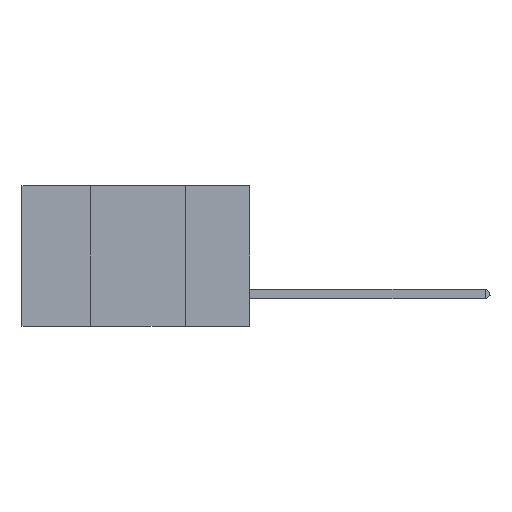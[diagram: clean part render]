
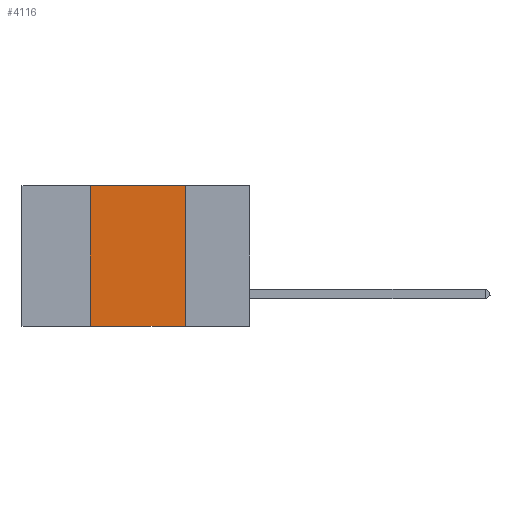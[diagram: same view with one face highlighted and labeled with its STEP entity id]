
A CAD part, left-side view. The second image highlights one B-rep face of the part: STEP entity #4116.
In plain terms, the highlighted planar face has unit normal (-1, 0, 0).
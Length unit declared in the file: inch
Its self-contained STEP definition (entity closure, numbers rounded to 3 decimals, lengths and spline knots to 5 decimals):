
#450 = EDGE_CURVE ( 'NONE', #1545, #4251, #6222, .T. ) ;
#472 = CARTESIAN_POINT ( 'NONE',  ( 0., 0.6, 0. ) ) ;
#520 = VECTOR ( 'NONE', #3350, 39.37008 ) ;
#592 = ORIENTED_EDGE ( 'NONE', *, *, #7883, .F. ) ;
#725 = VERTEX_POINT ( 'NONE', #2009 ) ;
#1063 = DIRECTION ( 'NONE',  ( 0., -1., 0. ) ) ;
#1291 = EDGE_LOOP ( 'NONE', ( #2982, #592, #4807, #7257 ) ) ;
#1545 = VERTEX_POINT ( 'NONE', #9071 ) ;
#2009 = CARTESIAN_POINT ( 'NONE',  ( 0., 0.17, -0.37 ) ) ;
#2027 = EDGE_CURVE ( 'NONE', #1545, #725, #5372, .T. ) ;
#2056 = AXIS2_PLACEMENT_3D ( 'NONE', #472, #8594, #6289 ) ;
#2134 = CARTESIAN_POINT ( 'NONE',  ( 0., 0.42, 0. ) ) ;
#2360 = EDGE_CURVE ( 'NONE', #4286, #725, #6974, .T. ) ;
#2982 = ORIENTED_EDGE ( 'NONE', *, *, #2360, .F. ) ;
#3350 = DIRECTION ( 'NONE',  ( 0., -1., 0. ) ) ;
#4076 = CARTESIAN_POINT ( 'NONE',  ( 0., 0.6, -0.37 ) ) ;
#4116 = ADVANCED_FACE ( 'NONE', ( #7621 ), #5554, .F. ) ;
#4251 = VERTEX_POINT ( 'NONE', #5859 ) ;
#4286 = VERTEX_POINT ( 'NONE', #8329 ) ;
#4652 = VECTOR ( 'NONE', #1063, 39.37008 ) ;
#4750 = VECTOR ( 'NONE', #7365, 39.37008 ) ;
#4807 = ORIENTED_EDGE ( 'NONE', *, *, #450, .F. ) ;
#5372 = LINE ( 'NONE', #4076, #520 ) ;
#5472 = VECTOR ( 'NONE', #7679, 39.37008 ) ;
#5554 = PLANE ( 'NONE',  #2056 ) ;
#5859 = CARTESIAN_POINT ( 'NONE',  ( 0., 0.42, 0. ) ) ;
#6141 = CARTESIAN_POINT ( 'NONE',  ( 0., 0.17, 0. ) ) ;
#6222 = LINE ( 'NONE', #2134, #4750 ) ;
#6289 = DIRECTION ( 'NONE',  ( 0., 0., -1. ) ) ;
#6610 = LINE ( 'NONE', #6963, #4652 ) ;
#6963 = CARTESIAN_POINT ( 'NONE',  ( 0., 0.6, 0. ) ) ;
#6974 = LINE ( 'NONE', #6141, #5472 ) ;
#7257 = ORIENTED_EDGE ( 'NONE', *, *, #2027, .T. ) ;
#7365 = DIRECTION ( 'NONE',  ( 0., 0., 1. ) ) ;
#7621 = FACE_OUTER_BOUND ( 'NONE', #1291, .T. ) ;
#7679 = DIRECTION ( 'NONE',  ( 0., 0., -1. ) ) ;
#7883 = EDGE_CURVE ( 'NONE', #4251, #4286, #6610, .T. ) ;
#8329 = CARTESIAN_POINT ( 'NONE',  ( 0., 0.17, 0. ) ) ;
#8594 = DIRECTION ( 'NONE',  ( 1., 0., 0. ) ) ;
#9071 = CARTESIAN_POINT ( 'NONE',  ( 0., 0.42, -0.37 ) ) ;
